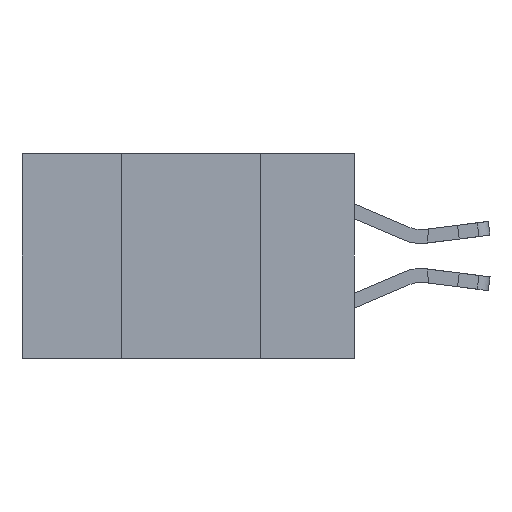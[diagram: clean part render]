
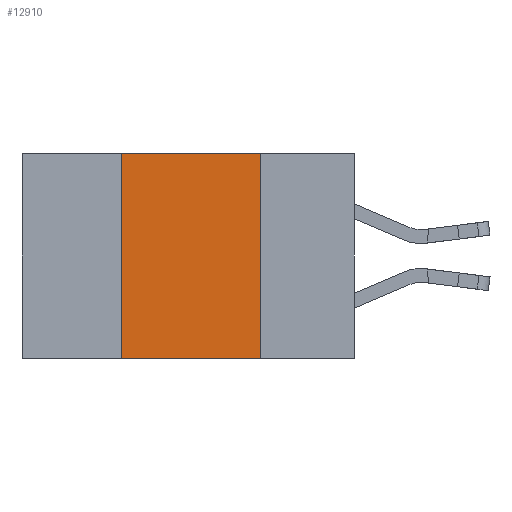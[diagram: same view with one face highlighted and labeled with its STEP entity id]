
A CAD part, left-side view. The second image highlights one B-rep face of the part: STEP entity #12910.
In plain terms, the highlighted planar face has unit normal (-1, 0, 0).
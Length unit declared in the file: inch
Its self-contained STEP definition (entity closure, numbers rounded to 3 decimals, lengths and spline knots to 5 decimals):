
#276 = FACE_OUTER_BOUND ( 'NONE', #22183, .T. ) ;
#1449 = VERTEX_POINT ( 'NONE', #21769 ) ;
#2517 = VERTEX_POINT ( 'NONE', #16692 ) ;
#2673 = ORIENTED_EDGE ( 'NONE', *, *, #9689, .F. ) ;
#3272 = LINE ( 'NONE', #20761, #20664 ) ;
#3382 = AXIS2_PLACEMENT_3D ( 'NONE', #9724, #21753, #11525 ) ;
#3878 = LINE ( 'NONE', #8939, #8568 ) ;
#4105 = ORIENTED_EDGE ( 'NONE', *, *, #16716, .F. ) ;
#4490 = EDGE_CURVE ( 'NONE', #18815, #5860, #3272, .T. ) ;
#5860 = VERTEX_POINT ( 'NONE', #17255 ) ;
#6919 = DIRECTION ( 'NONE',  ( 0., -1., 0. ) ) ;
#7319 = VECTOR ( 'NONE', #17527, 39.37008 ) ;
#8568 = VECTOR ( 'NONE', #19313, 39.37008 ) ;
#8852 = CARTESIAN_POINT ( 'NONE',  ( 0., 0.17, -0.37 ) ) ;
#8939 = CARTESIAN_POINT ( 'NONE',  ( 0., 0.6, 0. ) ) ;
#9689 = EDGE_CURVE ( 'NONE', #5860, #1449, #3878, .T. ) ;
#9724 = CARTESIAN_POINT ( 'NONE',  ( 0., 0.6, 0. ) ) ;
#11525 = DIRECTION ( 'NONE',  ( 0., 0., -1. ) ) ;
#12640 = ORIENTED_EDGE ( 'NONE', *, *, #4490, .F. ) ;
#12910 = ADVANCED_FACE ( 'NONE', ( #276 ), #20054, .F. ) ;
#13260 = LINE ( 'NONE', #15676, #13800 ) ;
#13800 = VECTOR ( 'NONE', #6919, 39.37008 ) ;
#13995 = DIRECTION ( 'NONE',  ( 0., 0., 1. ) ) ;
#15676 = CARTESIAN_POINT ( 'NONE',  ( 0., 0.6, -0.37 ) ) ;
#15884 = CARTESIAN_POINT ( 'NONE',  ( 0., 0.42, -0.37 ) ) ;
#16692 = CARTESIAN_POINT ( 'NONE',  ( 0., 0.17, -0.37 ) ) ;
#16716 = EDGE_CURVE ( 'NONE', #1449, #2517, #21102, .T. ) ;
#17255 = CARTESIAN_POINT ( 'NONE',  ( 0., 0.42, 0. ) ) ;
#17527 = DIRECTION ( 'NONE',  ( 0., 0., -1. ) ) ;
#18815 = VERTEX_POINT ( 'NONE', #15884 ) ;
#19313 = DIRECTION ( 'NONE',  ( 0., -1., 0. ) ) ;
#20054 = PLANE ( 'NONE',  #3382 ) ;
#20664 = VECTOR ( 'NONE', #13995, 39.37008 ) ;
#20761 = CARTESIAN_POINT ( 'NONE',  ( 0., 0.42, -0.37 ) ) ;
#21102 = LINE ( 'NONE', #8852, #7319 ) ;
#21691 = ORIENTED_EDGE ( 'NONE', *, *, #22322, .T. ) ;
#21753 = DIRECTION ( 'NONE',  ( 1., 0., 0. ) ) ;
#21769 = CARTESIAN_POINT ( 'NONE',  ( 0., 0.17, 0. ) ) ;
#22183 = EDGE_LOOP ( 'NONE', ( #4105, #2673, #12640, #21691 ) ) ;
#22322 = EDGE_CURVE ( 'NONE', #18815, #2517, #13260, .T. ) ;
